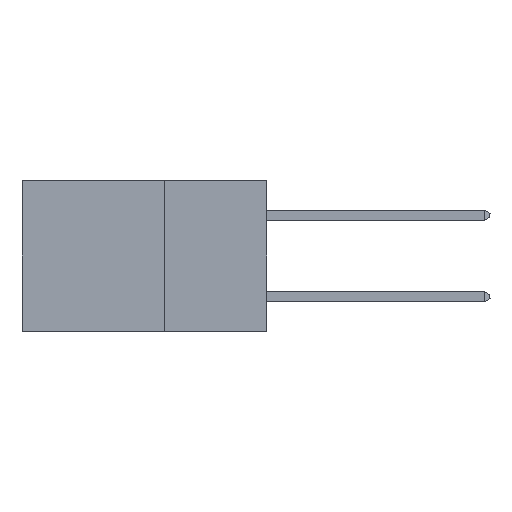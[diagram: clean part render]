
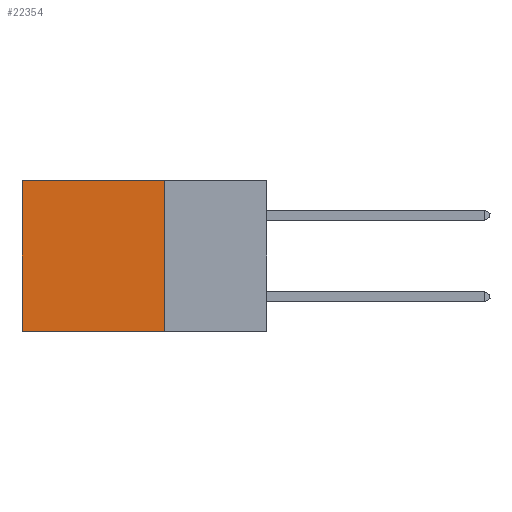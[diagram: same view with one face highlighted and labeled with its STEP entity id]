
A CAD part, left-side view. The second image highlights one B-rep face of the part: STEP entity #22354.
In plain terms, the highlighted planar face has unit normal (-1, 0, 0).
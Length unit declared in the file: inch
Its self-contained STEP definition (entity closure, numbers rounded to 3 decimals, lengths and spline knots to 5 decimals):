
#1522 = DIRECTION ( 'NONE',  ( 1., 0., 0. ) ) ;
#2252 = CARTESIAN_POINT ( 'NONE',  ( 0.2875, 0.6, -0.37 ) ) ;
#2956 = CARTESIAN_POINT ( 'NONE',  ( 0.2875, 0.25, 0. ) ) ;
#3352 = CARTESIAN_POINT ( 'NONE',  ( 0.2875, 0.25, 0. ) ) ;
#4678 = DIRECTION ( 'NONE',  ( 0., 0., -1. ) ) ;
#5744 = ORIENTED_EDGE ( 'NONE', *, *, #12208, .T. ) ;
#6293 = AXIS2_PLACEMENT_3D ( 'NONE', #17252, #1522, #17349 ) ;
#6407 = VECTOR ( 'NONE', #15139, 39.37008 ) ;
#6600 = LINE ( 'NONE', #3352, #13313 ) ;
#7478 = VECTOR ( 'NONE', #4678, 39.37008 ) ;
#7771 = EDGE_CURVE ( 'NONE', #14589, #27743, #24217, .T. ) ;
#8304 = PLANE ( 'NONE',  #6293 ) ;
#8898 = LINE ( 'NONE', #20315, #7478 ) ;
#9179 = ORIENTED_EDGE ( 'NONE', *, *, #27703, .F. ) ;
#9569 = ORIENTED_EDGE ( 'NONE', *, *, #7771, .F. ) ;
#9683 = CARTESIAN_POINT ( 'NONE',  ( 0.2875, 0.25, -0.37 ) ) ;
#11382 = ORIENTED_EDGE ( 'NONE', *, *, #24275, .T. ) ;
#12208 = EDGE_CURVE ( 'NONE', #15035, #27743, #20418, .T. ) ;
#13313 = VECTOR ( 'NONE', #25767, 39.37008 ) ;
#13423 = CARTESIAN_POINT ( 'NONE',  ( 0.2875, 0.6, 0. ) ) ;
#14589 = VERTEX_POINT ( 'NONE', #9683 ) ;
#15035 = VERTEX_POINT ( 'NONE', #13423 ) ;
#15139 = DIRECTION ( 'NONE',  ( 0., 1., 0. ) ) ;
#16876 = DIRECTION ( 'NONE',  ( 0., 0., -1. ) ) ;
#17252 = CARTESIAN_POINT ( 'NONE',  ( 0.2875, 0.25, 0. ) ) ;
#17349 = DIRECTION ( 'NONE',  ( 0., 0., -1. ) ) ;
#19720 = VECTOR ( 'NONE', #16876, 39.37008 ) ;
#19932 = FACE_OUTER_BOUND ( 'NONE', #22864, .T. ) ;
#20272 = VERTEX_POINT ( 'NONE', #2956 ) ;
#20315 = CARTESIAN_POINT ( 'NONE',  ( 0.2875, 0.25, 0. ) ) ;
#20418 = LINE ( 'NONE', #25684, #19720 ) ;
#22354 = ADVANCED_FACE ( 'NONE', ( #19932 ), #8304, .F. ) ;
#22864 = EDGE_LOOP ( 'NONE', ( #5744, #9569, #9179, #11382 ) ) ;
#24217 = LINE ( 'NONE', #28240, #6407 ) ;
#24275 = EDGE_CURVE ( 'NONE', #20272, #15035, #6600, .T. ) ;
#25684 = CARTESIAN_POINT ( 'NONE',  ( 0.2875, 0.6, 0. ) ) ;
#25767 = DIRECTION ( 'NONE',  ( 0., 1., 0. ) ) ;
#27703 = EDGE_CURVE ( 'NONE', #20272, #14589, #8898, .T. ) ;
#27743 = VERTEX_POINT ( 'NONE', #2252 ) ;
#28240 = CARTESIAN_POINT ( 'NONE',  ( 0.2875, 0.25, -0.37 ) ) ;
